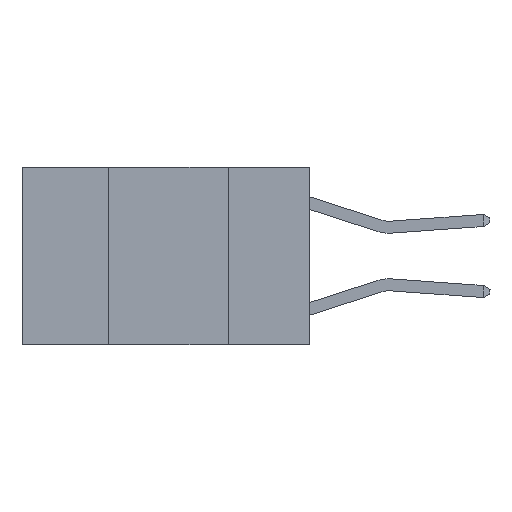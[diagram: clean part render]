
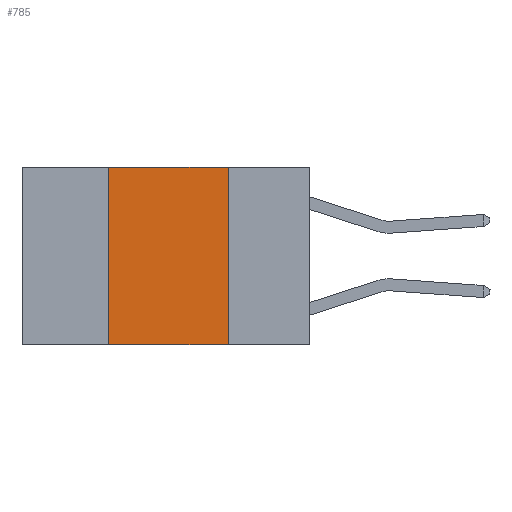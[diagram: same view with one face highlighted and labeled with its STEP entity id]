
A CAD part, left-side view. The second image highlights one B-rep face of the part: STEP entity #785.
In plain terms, the highlighted planar face has unit normal (-1, 0, 0).
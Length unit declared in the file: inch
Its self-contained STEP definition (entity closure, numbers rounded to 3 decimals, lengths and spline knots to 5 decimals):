
#160 = CARTESIAN_POINT ( 'NONE',  ( 0., 0.42, -0.37 ) ) ;
#207 = VECTOR ( 'NONE', #6447, 39.37008 ) ;
#358 = DIRECTION ( 'NONE',  ( 0., 0., -1. ) ) ;
#464 = EDGE_CURVE ( 'NONE', #3025, #3810, #5647, .T. ) ;
#472 = VECTOR ( 'NONE', #8400, 39.37008 ) ;
#785 = ADVANCED_FACE ( 'NONE', ( #2975 ), #2822, .F. ) ;
#897 = VERTEX_POINT ( 'NONE', #3267 ) ;
#1202 = AXIS2_PLACEMENT_3D ( 'NONE', #7434, #7263, #8532 ) ;
#1643 = EDGE_CURVE ( 'NONE', #897, #3810, #8489, .T. ) ;
#2256 = EDGE_LOOP ( 'NONE', ( #7816, #6352, #8643, #3516 ) ) ;
#2392 = LINE ( 'NONE', #7770, #472 ) ;
#2518 = CARTESIAN_POINT ( 'NONE',  ( 0., 0.42, 0. ) ) ;
#2743 = CARTESIAN_POINT ( 'NONE',  ( 0., 0.17, -0.37 ) ) ;
#2822 = PLANE ( 'NONE',  #1202 ) ;
#2975 = FACE_OUTER_BOUND ( 'NONE', #2256, .T. ) ;
#3025 = VERTEX_POINT ( 'NONE', #160 ) ;
#3267 = CARTESIAN_POINT ( 'NONE',  ( 0., 0.17, 0. ) ) ;
#3516 = ORIENTED_EDGE ( 'NONE', *, *, #464, .T. ) ;
#3810 = VERTEX_POINT ( 'NONE', #2743 ) ;
#4112 = VECTOR ( 'NONE', #6417, 39.37008 ) ;
#4752 = VERTEX_POINT ( 'NONE', #2518 ) ;
#5206 = CARTESIAN_POINT ( 'NONE',  ( 0., 0.6, -0.37 ) ) ;
#5235 = EDGE_CURVE ( 'NONE', #3025, #4752, #2392, .T. ) ;
#5647 = LINE ( 'NONE', #5206, #4112 ) ;
#5672 = LINE ( 'NONE', #5743, #207 ) ;
#5743 = CARTESIAN_POINT ( 'NONE',  ( 0., 0.6, 0. ) ) ;
#6352 = ORIENTED_EDGE ( 'NONE', *, *, #8540, .F. ) ;
#6417 = DIRECTION ( 'NONE',  ( 0., -1., 0. ) ) ;
#6447 = DIRECTION ( 'NONE',  ( 0., -1., 0. ) ) ;
#6710 = VECTOR ( 'NONE', #358, 39.37008 ) ;
#7263 = DIRECTION ( 'NONE',  ( 1., 0., 0. ) ) ;
#7434 = CARTESIAN_POINT ( 'NONE',  ( 0., 0.6, 0. ) ) ;
#7770 = CARTESIAN_POINT ( 'NONE',  ( 0., 0.42, 0. ) ) ;
#7816 = ORIENTED_EDGE ( 'NONE', *, *, #1643, .F. ) ;
#7831 = CARTESIAN_POINT ( 'NONE',  ( 0., 0.17, 0. ) ) ;
#8400 = DIRECTION ( 'NONE',  ( 0., 0., 1. ) ) ;
#8489 = LINE ( 'NONE', #7831, #6710 ) ;
#8532 = DIRECTION ( 'NONE',  ( 0., 0., -1. ) ) ;
#8540 = EDGE_CURVE ( 'NONE', #4752, #897, #5672, .T. ) ;
#8643 = ORIENTED_EDGE ( 'NONE', *, *, #5235, .F. ) ;
